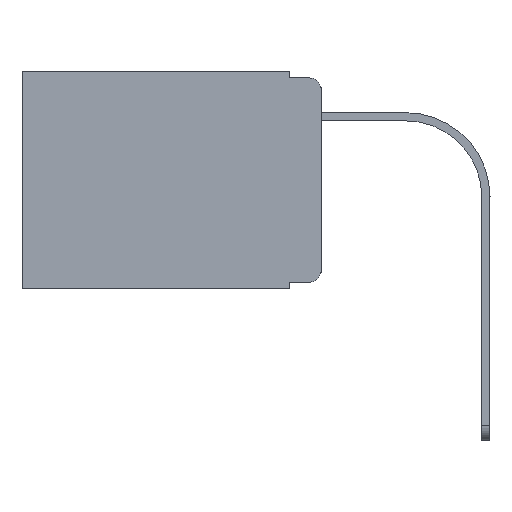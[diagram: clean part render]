
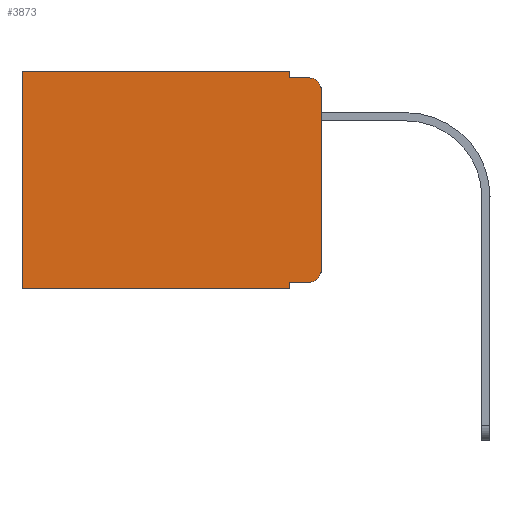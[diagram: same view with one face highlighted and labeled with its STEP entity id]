
A CAD part, left-side view. The second image highlights one B-rep face of the part: STEP entity #3873.
In plain terms, the highlighted planar face has unit normal (-1, 0, 0).
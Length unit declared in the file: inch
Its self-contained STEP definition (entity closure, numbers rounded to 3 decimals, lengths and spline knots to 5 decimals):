
#24 = VECTOR ( 'NONE', #12084, 39.37008 ) ;
#256 = VECTOR ( 'NONE', #13534, 39.37008 ) ;
#596 = AXIS2_PLACEMENT_3D ( 'NONE', #7820, #6724, #13745 ) ;
#1085 = FACE_OUTER_BOUND ( 'NONE', #11672, .T. ) ;
#1205 = ORIENTED_EDGE ( 'NONE', *, *, #7253, .F. ) ;
#1223 = ORIENTED_EDGE ( 'NONE', *, *, #2922, .T. ) ;
#1245 = DIRECTION ( 'NONE',  ( 0., 0., -1. ) ) ;
#1317 = LINE ( 'NONE', #6888, #256 ) ;
#1320 = CARTESIAN_POINT ( 'NONE',  ( 0.298, 0.051, -0.01 ) ) ;
#1717 = DIRECTION ( 'NONE',  ( 0., 0., -1. ) ) ;
#1867 = CARTESIAN_POINT ( 'NONE',  ( 0.298, 0.02, -0.333 ) ) ;
#2156 = CARTESIAN_POINT ( 'NONE',  ( 0.298, 0.473, -0.343 ) ) ;
#2254 = CARTESIAN_POINT ( 'NONE',  ( 0.298, 0.473, 0. ) ) ;
#2423 = VERTEX_POINT ( 'NONE', #3869 ) ;
#2922 = EDGE_CURVE ( 'NONE', #14132, #10178, #13204, .T. ) ;
#2950 = ORIENTED_EDGE ( 'NONE', *, *, #9895, .T. ) ;
#3454 = CARTESIAN_POINT ( 'NONE',  ( 0.298, 0., -0.03 ) ) ;
#3696 = DIRECTION ( 'NONE',  ( 0., 0., -1. ) ) ;
#3869 = CARTESIAN_POINT ( 'NONE',  ( 0.298, 0.02, -0.01 ) ) ;
#3873 = ADVANCED_FACE ( 'NONE', ( #1085 ), #12551, .F. ) ;
#4176 = EDGE_CURVE ( 'NONE', #13838, #8340, #5517, .T. ) ;
#4187 = LINE ( 'NONE', #7573, #24 ) ;
#4530 = ORIENTED_EDGE ( 'NONE', *, *, #12820, .T. ) ;
#4748 = LINE ( 'NONE', #2254, #9341 ) ;
#4858 = CIRCLE ( 'NONE', #14516, 0.02 ) ;
#4919 = CARTESIAN_POINT ( 'NONE',  ( 0.298, 0., -0.313 ) ) ;
#5027 = VERTEX_POINT ( 'NONE', #12385 ) ;
#5135 = LINE ( 'NONE', #10745, #8268 ) ;
#5494 = DIRECTION ( 'NONE',  ( 0., 0., -1. ) ) ;
#5517 = LINE ( 'NONE', #14506, #8183 ) ;
#6003 = CARTESIAN_POINT ( 'NONE',  ( 0.298, 0.473, 0. ) ) ;
#6161 = EDGE_CURVE ( 'NONE', #7482, #8340, #4748, .T. ) ;
#6314 = VECTOR ( 'NONE', #5494, 39.37008 ) ;
#6391 = ORIENTED_EDGE ( 'NONE', *, *, #14466, .F. ) ;
#6670 = DIRECTION ( 'NONE',  ( 0., -1., 0. ) ) ;
#6724 = DIRECTION ( 'NONE',  ( 1., 0., 0. ) ) ;
#6888 = CARTESIAN_POINT ( 'NONE',  ( 0.298, 0., 0. ) ) ;
#7253 = EDGE_CURVE ( 'NONE', #9179, #10178, #12280, .T. ) ;
#7415 = ORIENTED_EDGE ( 'NONE', *, *, #4176, .F. ) ;
#7482 = VERTEX_POINT ( 'NONE', #6003 ) ;
#7573 = CARTESIAN_POINT ( 'NONE',  ( 0.298, 0.051, 0. ) ) ;
#7751 = AXIS2_PLACEMENT_3D ( 'NONE', #8261, #13810, #3696 ) ;
#7820 = CARTESIAN_POINT ( 'NONE',  ( 0.298, 0., 0. ) ) ;
#8140 = EDGE_CURVE ( 'NONE', #11919, #7482, #1317, .T. ) ;
#8143 = ORIENTED_EDGE ( 'NONE', *, *, #13142, .F. ) ;
#8183 = VECTOR ( 'NONE', #12087, 39.37008 ) ;
#8261 = CARTESIAN_POINT ( 'NONE',  ( 0.298, 0.02, -0.313 ) ) ;
#8268 = VECTOR ( 'NONE', #1717, 39.37008 ) ;
#8340 = VERTEX_POINT ( 'NONE', #2156 ) ;
#8455 = CARTESIAN_POINT ( 'NONE',  ( 0.298, 0.051, -0.333 ) ) ;
#8756 = LINE ( 'NONE', #10964, #10819 ) ;
#8785 = EDGE_CURVE ( 'NONE', #11245, #13838, #4187, .T. ) ;
#8961 = CARTESIAN_POINT ( 'NONE',  ( 0.298, 0.051, 0. ) ) ;
#9172 = VECTOR ( 'NONE', #6670, 39.37008 ) ;
#9179 = VERTEX_POINT ( 'NONE', #3454 ) ;
#9341 = VECTOR ( 'NONE', #1245, 39.37008 ) ;
#9659 = CARTESIAN_POINT ( 'NONE',  ( 0.298, 0.02, -0.03 ) ) ;
#9895 = EDGE_CURVE ( 'NONE', #9179, #2423, #4858, .T. ) ;
#10019 = CARTESIAN_POINT ( 'NONE',  ( 0.298, 0.051, -0.343 ) ) ;
#10171 = ORIENTED_EDGE ( 'NONE', *, *, #6161, .T. ) ;
#10178 = VERTEX_POINT ( 'NONE', #4919 ) ;
#10701 = DIRECTION ( 'NONE',  ( -1., 0., 0. ) ) ;
#10745 = CARTESIAN_POINT ( 'NONE',  ( 0.298, 0.051, 0. ) ) ;
#10819 = VECTOR ( 'NONE', #13274, 39.37008 ) ;
#10964 = CARTESIAN_POINT ( 'NONE',  ( 0.298, 0.051, -0.333 ) ) ;
#11245 = VERTEX_POINT ( 'NONE', #8455 ) ;
#11672 = EDGE_LOOP ( 'NONE', ( #1205, #2950, #8143, #6391, #13912, #10171, #7415, #13575, #4530, #1223 ) ) ;
#11919 = VERTEX_POINT ( 'NONE', #8961 ) ;
#12084 = DIRECTION ( 'NONE',  ( 0., 0., -1. ) ) ;
#12087 = DIRECTION ( 'NONE',  ( 0., 1., 0. ) ) ;
#12130 = CARTESIAN_POINT ( 'NONE',  ( 0.298, 0., 0. ) ) ;
#12280 = LINE ( 'NONE', #12130, #6314 ) ;
#12385 = CARTESIAN_POINT ( 'NONE',  ( 0.298, 0.051, -0.01 ) ) ;
#12551 = PLANE ( 'NONE',  #596 ) ;
#12820 = EDGE_CURVE ( 'NONE', #11245, #14132, #8756, .T. ) ;
#13063 = DIRECTION ( 'NONE',  ( 0., 0., -1. ) ) ;
#13142 = EDGE_CURVE ( 'NONE', #5027, #2423, #13606, .T. ) ;
#13204 = CIRCLE ( 'NONE', #7751, 0.02 ) ;
#13274 = DIRECTION ( 'NONE',  ( 0., -1., 0. ) ) ;
#13534 = DIRECTION ( 'NONE',  ( 0., 1., 0. ) ) ;
#13575 = ORIENTED_EDGE ( 'NONE', *, *, #8785, .F. ) ;
#13606 = LINE ( 'NONE', #1320, #9172 ) ;
#13745 = DIRECTION ( 'NONE',  ( 0., 0., -1. ) ) ;
#13810 = DIRECTION ( 'NONE',  ( -1., 0., 0. ) ) ;
#13838 = VERTEX_POINT ( 'NONE', #10019 ) ;
#13912 = ORIENTED_EDGE ( 'NONE', *, *, #8140, .T. ) ;
#14132 = VERTEX_POINT ( 'NONE', #1867 ) ;
#14466 = EDGE_CURVE ( 'NONE', #11919, #5027, #5135, .T. ) ;
#14506 = CARTESIAN_POINT ( 'NONE',  ( 0.298, 0., -0.343 ) ) ;
#14516 = AXIS2_PLACEMENT_3D ( 'NONE', #9659, #10701, #13063 ) ;
